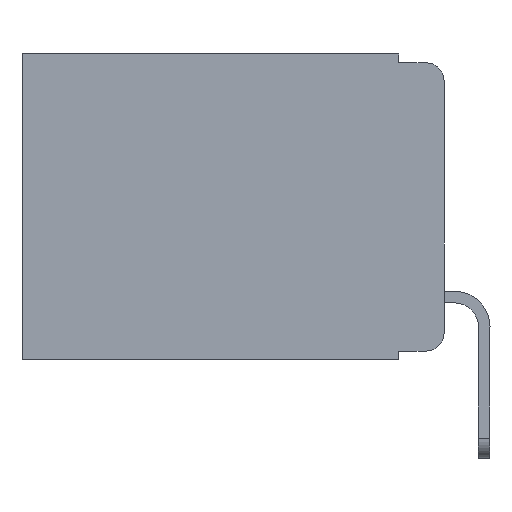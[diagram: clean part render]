
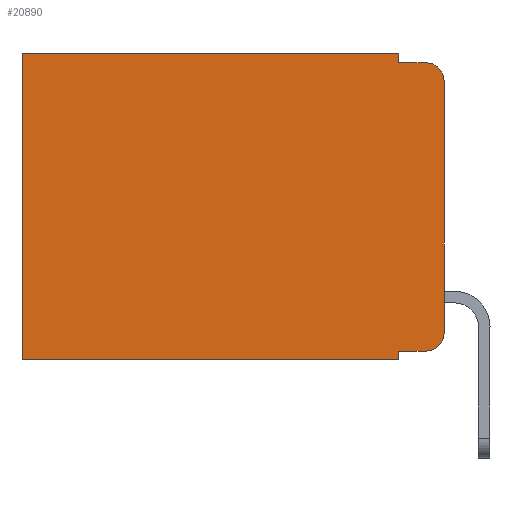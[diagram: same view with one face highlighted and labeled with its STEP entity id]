
A CAD part, left-side view. The second image highlights one B-rep face of the part: STEP entity #20890.
In plain terms, the highlighted planar face has unit normal (-1, 0, 0).
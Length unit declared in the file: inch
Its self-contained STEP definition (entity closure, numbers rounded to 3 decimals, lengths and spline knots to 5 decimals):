
#217 = CARTESIAN_POINT ( 'NONE',  ( 0.298, 0.051, 0. ) ) ;
#256 = CARTESIAN_POINT ( 'NONE',  ( 0.298, 0.02, -0.333 ) ) ;
#364 = VERTEX_POINT ( 'NONE', #21719 ) ;
#770 = EDGE_LOOP ( 'NONE', ( #9643, #11729, #8681, #4177, #10794, #10670, #15978, #15396, #8371, #4324 ) ) ;
#1940 = VERTEX_POINT ( 'NONE', #256 ) ;
#1971 = DIRECTION ( 'NONE',  ( 0., 0., -1. ) ) ;
#2267 = DIRECTION ( 'NONE',  ( 0., 1., 0. ) ) ;
#3164 = EDGE_CURVE ( 'NONE', #1940, #16073, #21357, .T. ) ;
#3374 = VERTEX_POINT ( 'NONE', #11273 ) ;
#3378 = LINE ( 'NONE', #4175, #10316 ) ;
#3534 = DIRECTION ( 'NONE',  ( -1., 0., 0. ) ) ;
#3599 = PLANE ( 'NONE',  #3700 ) ;
#3700 = AXIS2_PLACEMENT_3D ( 'NONE', #12759, #20229, #22068 ) ;
#4175 = CARTESIAN_POINT ( 'NONE',  ( 0.298, 0., 0. ) ) ;
#4177 = ORIENTED_EDGE ( 'NONE', *, *, #8465, .F. ) ;
#4324 = ORIENTED_EDGE ( 'NONE', *, *, #3164, .T. ) ;
#5895 = AXIS2_PLACEMENT_3D ( 'NONE', #13015, #3534, #14574 ) ;
#6379 = VERTEX_POINT ( 'NONE', #21995 ) ;
#6579 = CIRCLE ( 'NONE', #5895, 0.02 ) ;
#6919 = CARTESIAN_POINT ( 'NONE',  ( 0.298, 0.02, -0.01 ) ) ;
#8266 = LINE ( 'NONE', #13942, #23662 ) ;
#8283 = VERTEX_POINT ( 'NONE', #6919 ) ;
#8371 = ORIENTED_EDGE ( 'NONE', *, *, #17482, .T. ) ;
#8465 = EDGE_CURVE ( 'NONE', #14622, #364, #23896, .T. ) ;
#8681 = ORIENTED_EDGE ( 'NONE', *, *, #13427, .F. ) ;
#8859 = CARTESIAN_POINT ( 'NONE',  ( 0.298, 0.051, -0.01 ) ) ;
#9310 = AXIS2_PLACEMENT_3D ( 'NONE', #19419, #12025, #23215 ) ;
#9643 = ORIENTED_EDGE ( 'NONE', *, *, #12996, .F. ) ;
#10316 = VECTOR ( 'NONE', #17149, 39.37008 ) ;
#10670 = ORIENTED_EDGE ( 'NONE', *, *, #12373, .T. ) ;
#10794 = ORIENTED_EDGE ( 'NONE', *, *, #12990, .T. ) ;
#11221 = DIRECTION ( 'NONE',  ( 0., 0., -1. ) ) ;
#11273 = CARTESIAN_POINT ( 'NONE',  ( 0.298, 0.051, -0.333 ) ) ;
#11729 = ORIENTED_EDGE ( 'NONE', *, *, #23050, .T. ) ;
#11952 = CARTESIAN_POINT ( 'NONE',  ( 0.298, 0.051, -0.333 ) ) ;
#12025 = DIRECTION ( 'NONE',  ( -1., 0., 0. ) ) ;
#12169 = CARTESIAN_POINT ( 'NONE',  ( 0.298, 0.473, 0. ) ) ;
#12373 = EDGE_CURVE ( 'NONE', #13209, #14328, #13839, .T. ) ;
#12759 = CARTESIAN_POINT ( 'NONE',  ( 0.298, 0., 0. ) ) ;
#12917 = EDGE_CURVE ( 'NONE', #3374, #14343, #20233, .T. ) ;
#12990 = EDGE_CURVE ( 'NONE', #14622, #13209, #23394, .T. ) ;
#12996 = EDGE_CURVE ( 'NONE', #6379, #16073, #3378, .T. ) ;
#13015 = CARTESIAN_POINT ( 'NONE',  ( 0.298, 0.02, -0.03 ) ) ;
#13186 = CARTESIAN_POINT ( 'NONE',  ( 0.298, 0., 0. ) ) ;
#13209 = VERTEX_POINT ( 'NONE', #12169 ) ;
#13427 = EDGE_CURVE ( 'NONE', #364, #8283, #22211, .T. ) ;
#13839 = LINE ( 'NONE', #22439, #23123 ) ;
#13942 = CARTESIAN_POINT ( 'NONE',  ( 0.298, 0., -0.343 ) ) ;
#14010 = VECTOR ( 'NONE', #20613, 39.37008 ) ;
#14328 = VERTEX_POINT ( 'NONE', #22843 ) ;
#14343 = VERTEX_POINT ( 'NONE', #20826 ) ;
#14574 = DIRECTION ( 'NONE',  ( 0., 0., -1. ) ) ;
#14622 = VERTEX_POINT ( 'NONE', #16448 ) ;
#15050 = CARTESIAN_POINT ( 'NONE',  ( 0.298, 0.051, 0. ) ) ;
#15396 = ORIENTED_EDGE ( 'NONE', *, *, #12917, .F. ) ;
#15431 = CARTESIAN_POINT ( 'NONE',  ( 0.298, 0., -0.313 ) ) ;
#15798 = FACE_OUTER_BOUND ( 'NONE', #770, .T. ) ;
#15978 = ORIENTED_EDGE ( 'NONE', *, *, #24058, .F. ) ;
#16073 = VERTEX_POINT ( 'NONE', #15431 ) ;
#16138 = VECTOR ( 'NONE', #18272, 39.37008 ) ;
#16448 = CARTESIAN_POINT ( 'NONE',  ( 0.298, 0.051, 0. ) ) ;
#17149 = DIRECTION ( 'NONE',  ( 0., 0., -1. ) ) ;
#17333 = DIRECTION ( 'NONE',  ( 0., -1., 0. ) ) ;
#17482 = EDGE_CURVE ( 'NONE', #3374, #1940, #22982, .T. ) ;
#18272 = DIRECTION ( 'NONE',  ( 0., -1., 0. ) ) ;
#19419 = CARTESIAN_POINT ( 'NONE',  ( 0.298, 0.02, -0.313 ) ) ;
#19571 = DIRECTION ( 'NONE',  ( 0., 1., 0. ) ) ;
#19650 = VECTOR ( 'NONE', #11221, 39.37008 ) ;
#20208 = VECTOR ( 'NONE', #2267, 39.37008 ) ;
#20229 = DIRECTION ( 'NONE',  ( 1., 0., 0. ) ) ;
#20233 = LINE ( 'NONE', #15050, #19650 ) ;
#20613 = DIRECTION ( 'NONE',  ( 0., 0., -1. ) ) ;
#20826 = CARTESIAN_POINT ( 'NONE',  ( 0.298, 0.051, -0.343 ) ) ;
#20890 = ADVANCED_FACE ( 'NONE', ( #15798 ), #3599, .F. ) ;
#21237 = VECTOR ( 'NONE', #17333, 39.37008 ) ;
#21357 = CIRCLE ( 'NONE', #9310, 0.02 ) ;
#21719 = CARTESIAN_POINT ( 'NONE',  ( 0.298, 0.051, -0.01 ) ) ;
#21995 = CARTESIAN_POINT ( 'NONE',  ( 0.298, 0., -0.03 ) ) ;
#22068 = DIRECTION ( 'NONE',  ( 0., 0., -1. ) ) ;
#22211 = LINE ( 'NONE', #8859, #16138 ) ;
#22439 = CARTESIAN_POINT ( 'NONE',  ( 0.298, 0.473, 0. ) ) ;
#22843 = CARTESIAN_POINT ( 'NONE',  ( 0.298, 0.473, -0.343 ) ) ;
#22982 = LINE ( 'NONE', #11952, #21237 ) ;
#23050 = EDGE_CURVE ( 'NONE', #6379, #8283, #6579, .T. ) ;
#23123 = VECTOR ( 'NONE', #1971, 39.37008 ) ;
#23215 = DIRECTION ( 'NONE',  ( 0., 0., -1. ) ) ;
#23394 = LINE ( 'NONE', #13186, #20208 ) ;
#23662 = VECTOR ( 'NONE', #19571, 39.37008 ) ;
#23896 = LINE ( 'NONE', #217, #14010 ) ;
#24058 = EDGE_CURVE ( 'NONE', #14343, #14328, #8266, .T. ) ;
